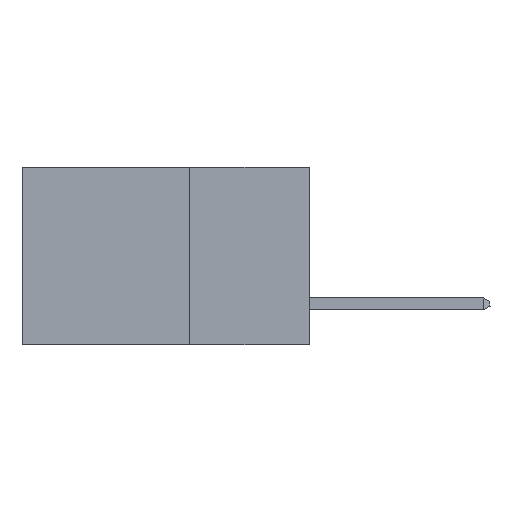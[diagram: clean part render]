
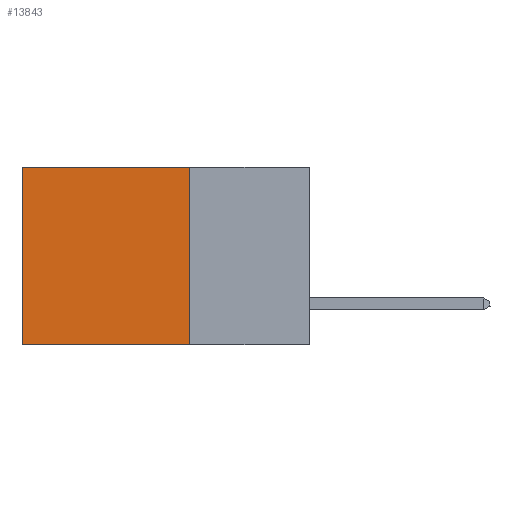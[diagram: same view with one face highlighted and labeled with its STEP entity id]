
A CAD part, left-side view. The second image highlights one B-rep face of the part: STEP entity #13843.
In plain terms, the highlighted planar face has unit normal (-1, 0, 0).
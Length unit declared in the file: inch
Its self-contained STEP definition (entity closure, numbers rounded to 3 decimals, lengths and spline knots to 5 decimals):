
#482 = CARTESIAN_POINT ( 'NONE',  ( 0.2875, 0.6, 0. ) ) ;
#1681 = LINE ( 'NONE', #14121, #2621 ) ;
#2543 = DIRECTION ( 'NONE',  ( 0., 0., -1. ) ) ;
#2547 = PLANE ( 'NONE',  #8923 ) ;
#2621 = VECTOR ( 'NONE', #14329, 39.37008 ) ;
#2875 = VERTEX_POINT ( 'NONE', #4880 ) ;
#3054 = CARTESIAN_POINT ( 'NONE',  ( 0.2875, 0.6, 0. ) ) ;
#3729 = CARTESIAN_POINT ( 'NONE',  ( 0.2875, 0.25, -0.37 ) ) ;
#4596 = LINE ( 'NONE', #12630, #6843 ) ;
#4761 = EDGE_LOOP ( 'NONE', ( #5240, #6397, #9040, #12546 ) ) ;
#4880 = CARTESIAN_POINT ( 'NONE',  ( 0.2875, 0.6, -0.37 ) ) ;
#5018 = LINE ( 'NONE', #3729, #13873 ) ;
#5155 = EDGE_CURVE ( 'NONE', #10201, #13201, #1681, .T. ) ;
#5240 = ORIENTED_EDGE ( 'NONE', *, *, #13373, .T. ) ;
#5356 = LINE ( 'NONE', #3054, #7605 ) ;
#5638 = DIRECTION ( 'NONE',  ( 0., 0., -1. ) ) ;
#6397 = ORIENTED_EDGE ( 'NONE', *, *, #12041, .F. ) ;
#6843 = VECTOR ( 'NONE', #5638, 39.37008 ) ;
#7292 = VERTEX_POINT ( 'NONE', #11704 ) ;
#7605 = VECTOR ( 'NONE', #2543, 39.37008 ) ;
#8709 = CARTESIAN_POINT ( 'NONE',  ( 0.2875, 0.25, 0. ) ) ;
#8923 = AXIS2_PLACEMENT_3D ( 'NONE', #8709, #14791, #13406 ) ;
#9040 = ORIENTED_EDGE ( 'NONE', *, *, #13305, .F. ) ;
#10201 = VERTEX_POINT ( 'NONE', #12022 ) ;
#11704 = CARTESIAN_POINT ( 'NONE',  ( 0.2875, 0.25, -0.37 ) ) ;
#12022 = CARTESIAN_POINT ( 'NONE',  ( 0.2875, 0.25, 0. ) ) ;
#12041 = EDGE_CURVE ( 'NONE', #7292, #2875, #5018, .T. ) ;
#12140 = DIRECTION ( 'NONE',  ( 0., 1., 0. ) ) ;
#12546 = ORIENTED_EDGE ( 'NONE', *, *, #5155, .T. ) ;
#12630 = CARTESIAN_POINT ( 'NONE',  ( 0.2875, 0.25, 0. ) ) ;
#13201 = VERTEX_POINT ( 'NONE', #482 ) ;
#13245 = FACE_OUTER_BOUND ( 'NONE', #4761, .T. ) ;
#13305 = EDGE_CURVE ( 'NONE', #10201, #7292, #4596, .T. ) ;
#13373 = EDGE_CURVE ( 'NONE', #13201, #2875, #5356, .T. ) ;
#13406 = DIRECTION ( 'NONE',  ( 0., 0., -1. ) ) ;
#13843 = ADVANCED_FACE ( 'NONE', ( #13245 ), #2547, .F. ) ;
#13873 = VECTOR ( 'NONE', #12140, 39.37008 ) ;
#14121 = CARTESIAN_POINT ( 'NONE',  ( 0.2875, 0.25, 0. ) ) ;
#14329 = DIRECTION ( 'NONE',  ( 0., 1., 0. ) ) ;
#14791 = DIRECTION ( 'NONE',  ( 1., 0., 0. ) ) ;
